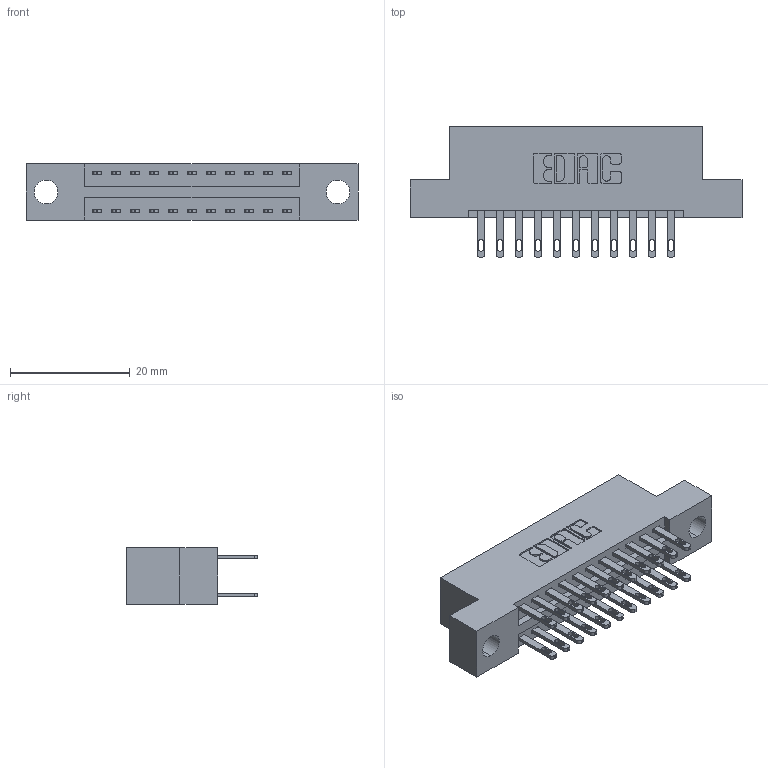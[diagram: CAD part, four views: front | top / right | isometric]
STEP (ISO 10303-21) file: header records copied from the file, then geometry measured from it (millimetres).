
FILE_DESCRIPTION (( 'STEP AP203' ), '1' );
FILE_NAME ('346-022-500-204.STEP', '2022-05-18T20:26:01', ( '' ), ( '' ), 'SwSTEP 2.0', 'SolidWorks 2020', '' );
FILE_SCHEMA (( 'CONFIG_CONTROL_DESIGN' ));
Length unit declared in the file: inch
Products named in the file (3): 346 Part_Flush Mounting Lugs - 0.156 Dia-TH; 346-022-500-204; 345-292-001_345-293-100
Assembly tree (23 placements, depth 2):
  346-022-500-204
    346 Part_Flush Mounting Lugs - 0.156 Dia-TH
    345-292-001_345-293-100  x22
Bounding box: 55.5 x 21.84 x 9.4 mm (x, y, z)
Volume: 5132.3 mm3; surface area: 6645.7 mm2
Topology: 23 solids, 23 shells, 1192 faces, 3599 edges, 2398 vertices
Faces by surface type: plane 728, cylinder 464
Entity records: 11701 total; most frequent: CARTESIAN_POINT 1974, ORIENTED_EDGE 1906, DIRECTION 1793, EDGE_CURVE 953, VECTOR 773, LINE 773, VERTEX_POINT 634, AXIS2_PLACEMENT_3D 510
